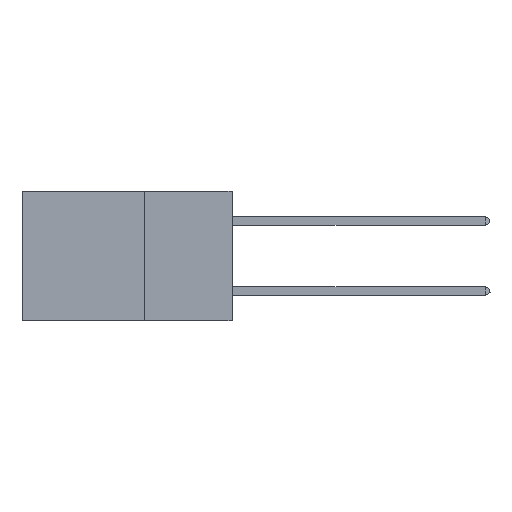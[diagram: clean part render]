
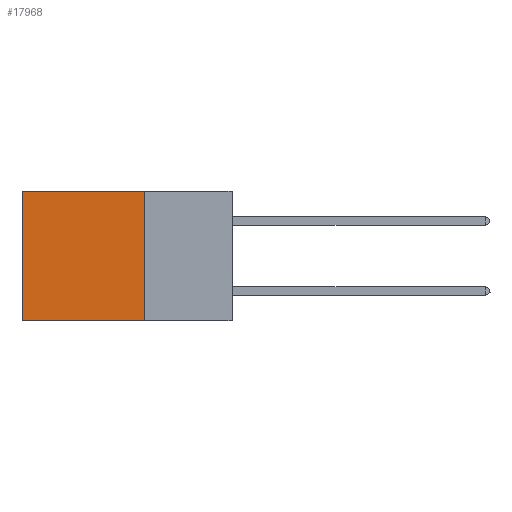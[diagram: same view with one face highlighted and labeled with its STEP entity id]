
A CAD part, left-side view. The second image highlights one B-rep face of the part: STEP entity #17968.
In plain terms, the highlighted planar face has unit normal (-1, 0, 0).
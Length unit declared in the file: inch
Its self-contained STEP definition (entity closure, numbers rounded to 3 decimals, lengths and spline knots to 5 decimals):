
#1179 = AXIS2_PLACEMENT_3D ( 'NONE', #21231, #25375, #6743 ) ;
#2733 = PLANE ( 'NONE',  #1179 ) ;
#3362 = FACE_OUTER_BOUND ( 'NONE', #21982, .T. ) ;
#4806 = CARTESIAN_POINT ( 'NONE',  ( 0.2875, 0.6, 0. ) ) ;
#5188 = DIRECTION ( 'NONE',  ( 0., 0., -1. ) ) ;
#6733 = LINE ( 'NONE', #24518, #8628 ) ;
#6743 = DIRECTION ( 'NONE',  ( 0., 0., -1. ) ) ;
#6885 = VECTOR ( 'NONE', #23596, 39.37008 ) ;
#6939 = DIRECTION ( 'NONE',  ( 0., 1., 0. ) ) ;
#7339 = CARTESIAN_POINT ( 'NONE',  ( 0.2875, 0.25, 0. ) ) ;
#8392 = VERTEX_POINT ( 'NONE', #4806 ) ;
#8628 = VECTOR ( 'NONE', #18635, 39.37008 ) ;
#11104 = VERTEX_POINT ( 'NONE', #14067 ) ;
#11741 = EDGE_CURVE ( 'NONE', #11104, #25532, #21150, .T. ) ;
#12163 = ORIENTED_EDGE ( 'NONE', *, *, #19820, .F. ) ;
#12681 = VECTOR ( 'NONE', #6939, 39.37008 ) ;
#13027 = EDGE_CURVE ( 'NONE', #8392, #14987, #18806, .T. ) ;
#14067 = CARTESIAN_POINT ( 'NONE',  ( 0.2875, 0.25, 0. ) ) ;
#14347 = ORIENTED_EDGE ( 'NONE', *, *, #13027, .T. ) ;
#14953 = ORIENTED_EDGE ( 'NONE', *, *, #22271, .T. ) ;
#14987 = VERTEX_POINT ( 'NONE', #18571 ) ;
#17284 = VECTOR ( 'NONE', #5188, 39.37008 ) ;
#17766 = ORIENTED_EDGE ( 'NONE', *, *, #11741, .F. ) ;
#17968 = ADVANCED_FACE ( 'NONE', ( #3362 ), #2733, .F. ) ;
#18571 = CARTESIAN_POINT ( 'NONE',  ( 0.2875, 0.6, -0.37 ) ) ;
#18635 = DIRECTION ( 'NONE',  ( 0., 1., 0. ) ) ;
#18733 = CARTESIAN_POINT ( 'NONE',  ( 0.2875, 0.25, 0. ) ) ;
#18806 = LINE ( 'NONE', #19691, #6885 ) ;
#19691 = CARTESIAN_POINT ( 'NONE',  ( 0.2875, 0.6, 0. ) ) ;
#19820 = EDGE_CURVE ( 'NONE', #25532, #14987, #6733, .T. ) ;
#21150 = LINE ( 'NONE', #7339, #17284 ) ;
#21231 = CARTESIAN_POINT ( 'NONE',  ( 0.2875, 0.25, 0. ) ) ;
#21982 = EDGE_LOOP ( 'NONE', ( #14347, #12163, #17766, #14953 ) ) ;
#22271 = EDGE_CURVE ( 'NONE', #11104, #8392, #24644, .T. ) ;
#23596 = DIRECTION ( 'NONE',  ( 0., 0., -1. ) ) ;
#24518 = CARTESIAN_POINT ( 'NONE',  ( 0.2875, 0.25, -0.37 ) ) ;
#24609 = CARTESIAN_POINT ( 'NONE',  ( 0.2875, 0.25, -0.37 ) ) ;
#24644 = LINE ( 'NONE', #18733, #12681 ) ;
#25375 = DIRECTION ( 'NONE',  ( 1., 0., 0. ) ) ;
#25532 = VERTEX_POINT ( 'NONE', #24609 ) ;
